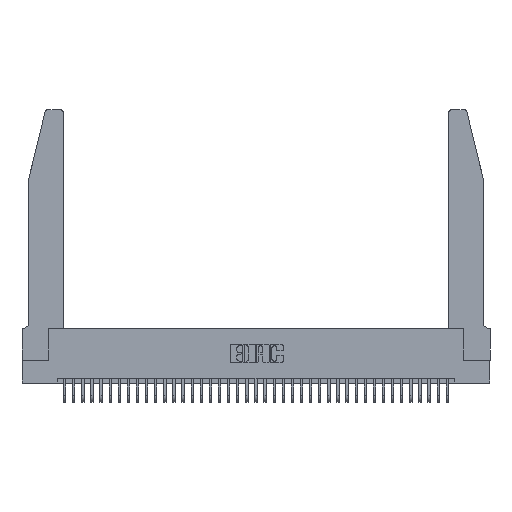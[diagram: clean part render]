
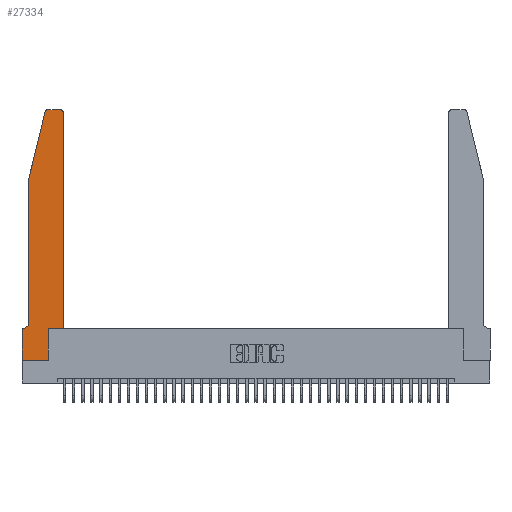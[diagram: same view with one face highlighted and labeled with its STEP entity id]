
A CAD part, top view. The second image highlights one B-rep face of the part: STEP entity #27334.
In plain terms, the highlighted planar face has unit normal (0, 0, 1).
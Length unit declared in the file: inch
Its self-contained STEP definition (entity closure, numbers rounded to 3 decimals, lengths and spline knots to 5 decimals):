
#319 = CARTESIAN_POINT ( 'NONE',  ( 0.2865, 0.35, 0.37 ) ) ;
#751 = PLANE ( 'NONE',  #1192 ) ;
#962 = LINE ( 'NONE', #30864, #32018 ) ;
#1192 = AXIS2_PLACEMENT_3D ( 'NONE', #10271, #31810, #13407 ) ;
#2019 = CARTESIAN_POINT ( 'NONE',  ( 0.4505, 2.72, 0.37 ) ) ;
#2213 = VECTOR ( 'NONE', #38048, 39.37008 ) ;
#2622 = VERTEX_POINT ( 'NONE', #19846 ) ;
#2639 = CARTESIAN_POINT ( 'NONE',  ( 0., 0., 0.37 ) ) ;
#2916 = ORIENTED_EDGE ( 'NONE', *, *, #23580, .T. ) ;
#3890 = EDGE_CURVE ( 'NONE', #22805, #38745, #19176, .T. ) ;
#3924 = ORIENTED_EDGE ( 'NONE', *, *, #37315, .T. ) ;
#3997 = LINE ( 'NONE', #18277, #27734 ) ;
#4665 = CARTESIAN_POINT ( 'NONE',  ( 0.0755, 2., 0.37 ) ) ;
#5836 = VERTEX_POINT ( 'NONE', #2639 ) ;
#6883 = LINE ( 'NONE', #36758, #14196 ) ;
#8364 = CARTESIAN_POINT ( 'NONE',  ( 0.0755, 0.35, 0.37 ) ) ;
#8419 = CARTESIAN_POINT ( 'NONE',  ( 0.284, 2.72, 0.37 ) ) ;
#8622 = EDGE_CURVE ( 'NONE', #11450, #35742, #25478, .T. ) ;
#8831 = CARTESIAN_POINT ( 'NONE',  ( 0.0055, 0.35, 0.37 ) ) ;
#9619 = VECTOR ( 'NONE', #29133, 39.37008 ) ;
#9839 = CARTESIAN_POINT ( 'NONE',  ( 0., 0.35, 0.37 ) ) ;
#10271 = CARTESIAN_POINT ( 'NONE',  ( 0., 0.35, 0.37 ) ) ;
#10279 = VERTEX_POINT ( 'NONE', #8831 ) ;
#11450 = VERTEX_POINT ( 'NONE', #2019 ) ;
#11539 = DIRECTION ( 'NONE',  ( 1., 0., 0. ) ) ;
#11575 = LINE ( 'NONE', #29809, #9619 ) ;
#12263 = ORIENTED_EDGE ( 'NONE', *, *, #27042, .T. ) ;
#12683 = EDGE_CURVE ( 'NONE', #14859, #17716, #29513, .T. ) ;
#12695 = CARTESIAN_POINT ( 'NONE',  ( 0.0755, 2., 0.37 ) ) ;
#12944 = VECTOR ( 'NONE', #23268, 39.37008 ) ;
#13086 = CARTESIAN_POINT ( 'NONE',  ( 0.0055, 0.42, 0.37 ) ) ;
#13407 = DIRECTION ( 'NONE',  ( 1., 0., 0. ) ) ;
#14196 = VECTOR ( 'NONE', #33715, 39.37008 ) ;
#14710 = EDGE_CURVE ( 'NONE', #14904, #2622, #3997, .T. ) ;
#14821 = EDGE_CURVE ( 'NONE', #35742, #22805, #962, .T. ) ;
#14859 = VERTEX_POINT ( 'NONE', #12695 ) ;
#14904 = VERTEX_POINT ( 'NONE', #319 ) ;
#16014 = VERTEX_POINT ( 'NONE', #39072 ) ;
#16127 = ORIENTED_EDGE ( 'NONE', *, *, #8622, .T. ) ;
#16212 = DIRECTION ( 'NONE',  ( -1., 0., 0. ) ) ;
#16660 = CARTESIAN_POINT ( 'NONE',  ( 0.4505, 0.35, 0.37 ) ) ;
#17716 = VERTEX_POINT ( 'NONE', #22844 ) ;
#18195 = DIRECTION ( 'NONE',  ( 0., 0., 1. ) ) ;
#18277 = CARTESIAN_POINT ( 'NONE',  ( 0.4505, 0.35, 0.37 ) ) ;
#18716 = LINE ( 'NONE', #35698, #34057 ) ;
#19176 = CIRCLE ( 'NONE', #20924, 0.03 ) ;
#19545 = CARTESIAN_POINT ( 'NONE',  ( 0.284, 2.75, 0.37 ) ) ;
#19846 = CARTESIAN_POINT ( 'NONE',  ( 0.4505, 0.35, 0.37 ) ) ;
#20924 = AXIS2_PLACEMENT_3D ( 'NONE', #8419, #30000, #11539 ) ;
#21186 = LINE ( 'NONE', #38348, #12944 ) ;
#21371 = DIRECTION ( 'NONE',  ( 1., 0., 0. ) ) ;
#21444 = ORIENTED_EDGE ( 'NONE', *, *, #3890, .T. ) ;
#22005 = EDGE_LOOP ( 'NONE', ( #31459, #21444, #23365, #37232, #31044, #35839, #12263, #28672, #2916, #27662, #3924, #16127 ) ) ;
#22329 = VECTOR ( 'NONE', #26351, 39.37008 ) ;
#22805 = VERTEX_POINT ( 'NONE', #19545 ) ;
#22844 = CARTESIAN_POINT ( 'NONE',  ( 0.0755, 0.42, 0.37 ) ) ;
#23268 = DIRECTION ( 'NONE',  ( 1., 0., 0. ) ) ;
#23365 = ORIENTED_EDGE ( 'NONE', *, *, #25400, .T. ) ;
#23580 = EDGE_CURVE ( 'NONE', #16014, #14904, #11575, .T. ) ;
#23790 = DIRECTION ( 'NONE',  ( -1., 0., 0. ) ) ;
#25010 = AXIS2_PLACEMENT_3D ( 'NONE', #13086, #34582, #16212 ) ;
#25400 = EDGE_CURVE ( 'NONE', #38745, #14859, #18716, .T. ) ;
#25478 = CIRCLE ( 'NONE', #34128, 0.03 ) ;
#26172 = LINE ( 'NONE', #8364, #33328 ) ;
#26351 = DIRECTION ( 'NONE',  ( 0., -1., 0. ) ) ;
#27042 = EDGE_CURVE ( 'NONE', #33284, #5836, #6883, .T. ) ;
#27334 = ADVANCED_FACE ( 'NONE', ( #28150 ), #751, .T. ) ;
#27662 = ORIENTED_EDGE ( 'NONE', *, *, #14710, .T. ) ;
#27734 = VECTOR ( 'NONE', #21371, 39.37008 ) ;
#27733 = CARTESIAN_POINT ( 'NONE',  ( 0.25487, 2.72718, 0.37 ) ) ;
#28150 = FACE_OUTER_BOUND ( 'NONE', #22005, .T. ) ;
#28672 = ORIENTED_EDGE ( 'NONE', *, *, #32946, .T. ) ;
#29133 = DIRECTION ( 'NONE',  ( 0., 1., 0. ) ) ;
#29423 = DIRECTION ( 'NONE',  ( -0.239, -0.971, 0. ) ) ;
#29513 = LINE ( 'NONE', #4665, #22329 ) ;
#29809 = CARTESIAN_POINT ( 'NONE',  ( 0.2865, 0.35, 0.37 ) ) ;
#30000 = DIRECTION ( 'NONE',  ( 0., 0., 1. ) ) ;
#30864 = CARTESIAN_POINT ( 'NONE',  ( 0.2605, 2.75, 0.37 ) ) ;
#30995 = DIRECTION ( 'NONE',  ( -1., 0., 0. ) ) ;
#31044 = ORIENTED_EDGE ( 'NONE', *, *, #32071, .T. ) ;
#31459 = ORIENTED_EDGE ( 'NONE', *, *, #14821, .T. ) ;
#31810 = DIRECTION ( 'NONE',  ( 0., 0., 1. ) ) ;
#32018 = VECTOR ( 'NONE', #30995, 39.37008 ) ;
#32071 = EDGE_CURVE ( 'NONE', #17716, #10279, #35075, .T. ) ;
#32946 = EDGE_CURVE ( 'NONE', #5836, #16014, #21186, .T. ) ;
#33284 = VERTEX_POINT ( 'NONE', #9839 ) ;
#33328 = VECTOR ( 'NONE', #23790, 39.37008 ) ;
#33715 = DIRECTION ( 'NONE',  ( 0., -1., 0. ) ) ;
#34057 = VECTOR ( 'NONE', #29423, 39.37008 ) ;
#34128 = AXIS2_PLACEMENT_3D ( 'NONE', #36515, #18195, #39556 ) ;
#34160 = LINE ( 'NONE', #16660, #2213 ) ;
#34582 = DIRECTION ( 'NONE',  ( 0., 0., -1. ) ) ;
#34824 = EDGE_CURVE ( 'NONE', #10279, #33284, #26172, .T. ) ;
#35075 = CIRCLE ( 'NONE', #25010, 0.07 ) ;
#35698 = CARTESIAN_POINT ( 'NONE',  ( 0.0755, 2., 0.37 ) ) ;
#35742 = VERTEX_POINT ( 'NONE', #36182 ) ;
#35839 = ORIENTED_EDGE ( 'NONE', *, *, #34824, .T. ) ;
#36182 = CARTESIAN_POINT ( 'NONE',  ( 0.4205, 2.75, 0.37 ) ) ;
#36515 = CARTESIAN_POINT ( 'NONE',  ( 0.4205, 2.72, 0.37 ) ) ;
#36758 = CARTESIAN_POINT ( 'NONE',  ( 0., 0., 0.37 ) ) ;
#37232 = ORIENTED_EDGE ( 'NONE', *, *, #12683, .T. ) ;
#37315 = EDGE_CURVE ( 'NONE', #2622, #11450, #34160, .T. ) ;
#38048 = DIRECTION ( 'NONE',  ( 0., 1., 0. ) ) ;
#38348 = CARTESIAN_POINT ( 'NONE',  ( 0., 0., 0.37 ) ) ;
#38745 = VERTEX_POINT ( 'NONE', #27733 ) ;
#39072 = CARTESIAN_POINT ( 'NONE',  ( 0.2865, 0., 0.37 ) ) ;
#39556 = DIRECTION ( 'NONE',  ( 1., 0., 0. ) ) ;
